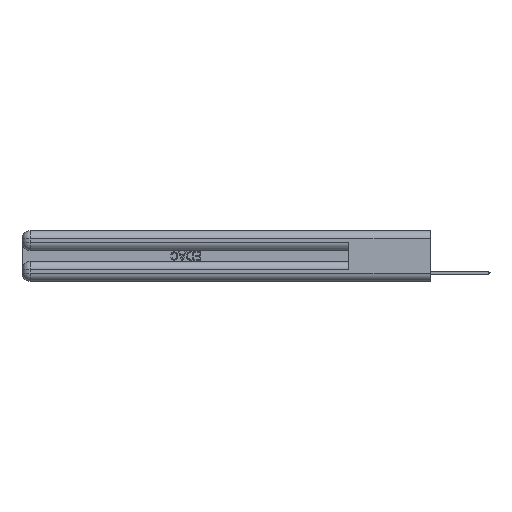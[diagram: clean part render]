
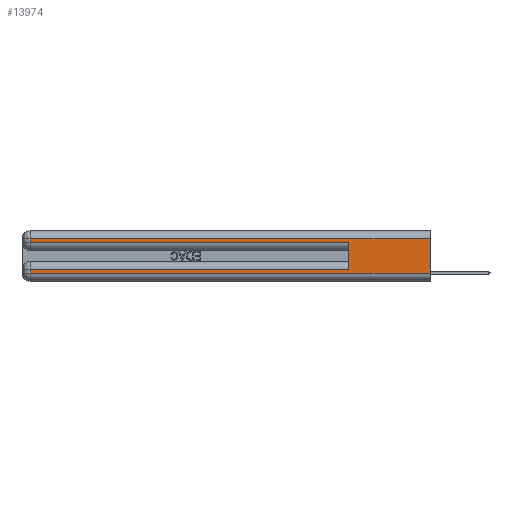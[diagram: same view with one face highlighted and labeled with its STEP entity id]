
A CAD part, left-side view. The second image highlights one B-rep face of the part: STEP entity #13974.
In plain terms, the highlighted planar face has unit normal (-1, 0, 0).
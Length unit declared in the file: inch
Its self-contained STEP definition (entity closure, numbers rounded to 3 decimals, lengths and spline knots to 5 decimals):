
#230 = CARTESIAN_POINT ( 'NONE',  ( 0., 2.94, 0.06 ) ) ;
#552 = VERTEX_POINT ( 'NONE', #21352 ) ;
#697 = CARTESIAN_POINT ( 'NONE',  ( 0., 0.6, 0.085 ) ) ;
#1780 = ORIENTED_EDGE ( 'NONE', *, *, #5413, .F. ) ;
#1888 = FACE_OUTER_BOUND ( 'NONE', #16238, .T. ) ;
#2866 = VERTEX_POINT ( 'NONE', #697 ) ;
#3315 = DIRECTION ( 'NONE',  ( 0., 1., 0. ) ) ;
#3444 = CARTESIAN_POINT ( 'NONE',  ( 0., 0., 0.06 ) ) ;
#3739 = VERTEX_POINT ( 'NONE', #18835 ) ;
#4679 = ORIENTED_EDGE ( 'NONE', *, *, #7371, .T. ) ;
#4774 = VERTEX_POINT ( 'NONE', #19498 ) ;
#5413 = EDGE_CURVE ( 'NONE', #2866, #552, #19419, .T. ) ;
#6390 = ORIENTED_EDGE ( 'NONE', *, *, #19398, .T. ) ;
#6764 = AXIS2_PLACEMENT_3D ( 'NONE', #6769, #32980, #22742 ) ;
#6769 = CARTESIAN_POINT ( 'NONE',  ( 0., 0., 0.37 ) ) ;
#7371 = EDGE_CURVE ( 'NONE', #15835, #12068, #11898, .T. ) ;
#8373 = EDGE_CURVE ( 'NONE', #2866, #15835, #22994, .T. ) ;
#8532 = EDGE_CURVE ( 'NONE', #25216, #4774, #18495, .T. ) ;
#8653 = DIRECTION ( 'NONE',  ( 0., 0., 1. ) ) ;
#9599 = PLANE ( 'NONE',  #6764 ) ;
#10721 = VECTOR ( 'NONE', #15363, 39.37008 ) ;
#11372 = CARTESIAN_POINT ( 'NONE',  ( 0., 2.94, 0.31 ) ) ;
#11718 = LINE ( 'NONE', #16601, #32523 ) ;
#11753 = LINE ( 'NONE', #33342, #20744 ) ;
#11859 = EDGE_CURVE ( 'NONE', #4774, #552, #11753, .T. ) ;
#11898 = LINE ( 'NONE', #12124, #22526 ) ;
#12068 = VERTEX_POINT ( 'NONE', #230 ) ;
#12124 = CARTESIAN_POINT ( 'NONE',  ( 0., 2.94, 0.37 ) ) ;
#13162 = ORIENTED_EDGE ( 'NONE', *, *, #8373, .T. ) ;
#13544 = DIRECTION ( 'NONE',  ( 0., -1., 0. ) ) ;
#13974 = ADVANCED_FACE ( 'NONE', ( #1888 ), #9599, .F. ) ;
#15363 = DIRECTION ( 'NONE',  ( 0., 0., -1. ) ) ;
#15835 = VERTEX_POINT ( 'NONE', #22854 ) ;
#15899 = ORIENTED_EDGE ( 'NONE', *, *, #20036, .F. ) ;
#16035 = LINE ( 'NONE', #26496, #31530 ) ;
#16238 = EDGE_LOOP ( 'NONE', ( #15899, #32973, #28595, #24987, #1780, #13162, #4679, #6390 ) ) ;
#16601 = CARTESIAN_POINT ( 'NONE',  ( 0., 0., 0.31 ) ) ;
#17278 = VECTOR ( 'NONE', #13544, 39.37008 ) ;
#17654 = LINE ( 'NONE', #3444, #17278 ) ;
#18495 = LINE ( 'NONE', #30967, #10721 ) ;
#18835 = CARTESIAN_POINT ( 'NONE',  ( 0., 0., 0.06 ) ) ;
#19398 = EDGE_CURVE ( 'NONE', #12068, #3739, #17654, .T. ) ;
#19419 = LINE ( 'NONE', #26801, #23900 ) ;
#19498 = CARTESIAN_POINT ( 'NONE',  ( 0., 2.94, 0.285 ) ) ;
#19606 = DIRECTION ( 'NONE',  ( 0., 1., 0. ) ) ;
#19828 = CARTESIAN_POINT ( 'NONE',  ( 0., 0., 0.085 ) ) ;
#20013 = DIRECTION ( 'NONE',  ( 0., 0., -1. ) ) ;
#20036 = EDGE_CURVE ( 'NONE', #31519, #3739, #16035, .T. ) ;
#20744 = VECTOR ( 'NONE', #20808, 39.37008 ) ;
#20808 = DIRECTION ( 'NONE',  ( 0., -1., 0. ) ) ;
#21352 = CARTESIAN_POINT ( 'NONE',  ( 0., 0.6, 0.285 ) ) ;
#22526 = VECTOR ( 'NONE', #20013, 39.37008 ) ;
#22604 = EDGE_CURVE ( 'NONE', #31519, #25216, #11718, .T. ) ;
#22742 = DIRECTION ( 'NONE',  ( 0., 0., -1. ) ) ;
#22854 = CARTESIAN_POINT ( 'NONE',  ( 0., 2.94, 0.085 ) ) ;
#22994 = LINE ( 'NONE', #19828, #31971 ) ;
#23885 = DIRECTION ( 'NONE',  ( 0., 0., -1. ) ) ;
#23900 = VECTOR ( 'NONE', #8653, 39.37008 ) ;
#24987 = ORIENTED_EDGE ( 'NONE', *, *, #11859, .T. ) ;
#25216 = VERTEX_POINT ( 'NONE', #11372 ) ;
#26496 = CARTESIAN_POINT ( 'NONE',  ( 0., 0., 0.37 ) ) ;
#26801 = CARTESIAN_POINT ( 'NONE',  ( 0., 0.6, 0.145 ) ) ;
#28595 = ORIENTED_EDGE ( 'NONE', *, *, #8532, .T. ) ;
#30967 = CARTESIAN_POINT ( 'NONE',  ( 0., 2.94, 0.37 ) ) ;
#31519 = VERTEX_POINT ( 'NONE', #32575 ) ;
#31530 = VECTOR ( 'NONE', #23885, 39.37008 ) ;
#31971 = VECTOR ( 'NONE', #19606, 39.37008 ) ;
#32523 = VECTOR ( 'NONE', #3315, 39.37008 ) ;
#32575 = CARTESIAN_POINT ( 'NONE',  ( 0., 0., 0.31 ) ) ;
#32973 = ORIENTED_EDGE ( 'NONE', *, *, #22604, .T. ) ;
#32980 = DIRECTION ( 'NONE',  ( 1., 0., 0. ) ) ;
#33342 = CARTESIAN_POINT ( 'NONE',  ( 0., 0., 0.285 ) ) ;
